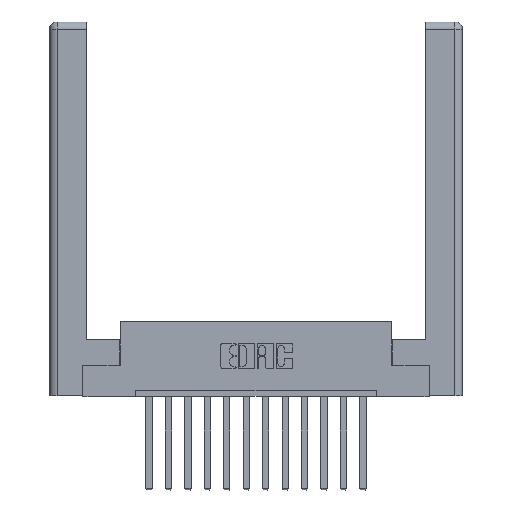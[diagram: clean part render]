
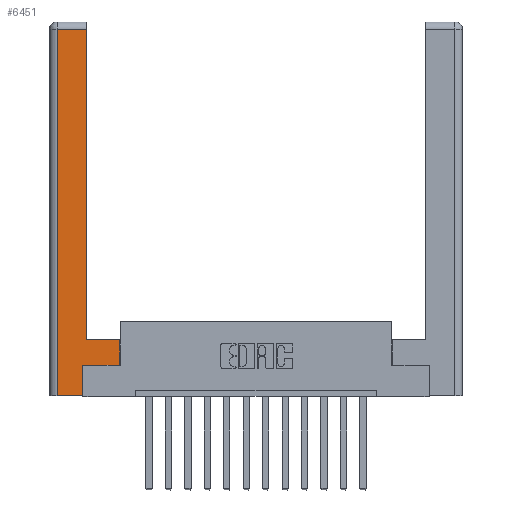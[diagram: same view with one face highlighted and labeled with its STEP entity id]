
A CAD part, top view. The second image highlights one B-rep face of the part: STEP entity #6451.
In plain terms, the highlighted planar face has unit normal (0, 0, 1).
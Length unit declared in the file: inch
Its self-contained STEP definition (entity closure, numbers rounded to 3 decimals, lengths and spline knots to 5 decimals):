
#44 = EDGE_CURVE ( 'NONE', #8756, #13986, #4058, .T. ) ;
#357 = DIRECTION ( 'NONE',  ( -1., 0., 0. ) ) ;
#538 = ORIENTED_EDGE ( 'NONE', *, *, #11361, .T. ) ;
#880 = DIRECTION ( 'NONE',  ( 0., -1., 0. ) ) ;
#919 = CARTESIAN_POINT ( 'NONE',  ( 0.265, 0., 0. ) ) ;
#1040 = VECTOR ( 'NONE', #12653, 39.37008 ) ;
#1096 = VERTEX_POINT ( 'NONE', #3537 ) ;
#1991 = CARTESIAN_POINT ( 'NONE',  ( 0.295, 2.94, 0. ) ) ;
#2086 = EDGE_CURVE ( 'NONE', #8800, #8756, #11748, .T. ) ;
#2091 = LINE ( 'NONE', #3829, #6726 ) ;
#2126 = EDGE_CURVE ( 'NONE', #13986, #3069, #9724, .T. ) ;
#2316 = VECTOR ( 'NONE', #14086, 39.37008 ) ;
#3002 = CARTESIAN_POINT ( 'NONE',  ( 0.0615, 2.94, 0. ) ) ;
#3069 = VERTEX_POINT ( 'NONE', #10200 ) ;
#3183 = ORIENTED_EDGE ( 'NONE', *, *, #6002, .T. ) ;
#3537 = CARTESIAN_POINT ( 'NONE',  ( 0.565, 0.245, 0. ) ) ;
#3702 = VERTEX_POINT ( 'NONE', #1991 ) ;
#3773 = ORIENTED_EDGE ( 'NONE', *, *, #44, .T. ) ;
#3806 = EDGE_CURVE ( 'NONE', #14374, #13888, #2091, .T. ) ;
#3829 = CARTESIAN_POINT ( 'NONE',  ( 0.295, 0.45, 0. ) ) ;
#3985 = PLANE ( 'NONE',  #7229 ) ;
#4058 = LINE ( 'NONE', #919, #9979 ) ;
#4127 = CARTESIAN_POINT ( 'NONE',  ( 0.0615, 0., 0. ) ) ;
#5360 = ORIENTED_EDGE ( 'NONE', *, *, #6466, .T. ) ;
#5579 = ORIENTED_EDGE ( 'NONE', *, *, #2086, .T. ) ;
#5598 = CARTESIAN_POINT ( 'NONE',  ( 0.0615, 0., 0. ) ) ;
#5719 = ORIENTED_EDGE ( 'NONE', *, *, #2126, .T. ) ;
#5774 = DIRECTION ( 'NONE',  ( 1., 0., 0. ) ) ;
#6002 = EDGE_CURVE ( 'NONE', #13888, #3702, #13449, .T. ) ;
#6110 = CARTESIAN_POINT ( 'NONE',  ( 0.565, 0.45, 0. ) ) ;
#6266 = VECTOR ( 'NONE', #14195, 39.37008 ) ;
#6352 = DIRECTION ( 'NONE',  ( 0., 0., -1. ) ) ;
#6451 = ADVANCED_FACE ( 'NONE', ( #6616 ), #3985, .F. ) ;
#6466 = EDGE_CURVE ( 'NONE', #3702, #8800, #12165, .T. ) ;
#6616 = FACE_OUTER_BOUND ( 'NONE', #12034, .T. ) ;
#6726 = VECTOR ( 'NONE', #357, 39.37008 ) ;
#7229 = AXIS2_PLACEMENT_3D ( 'NONE', #11104, #6352, #10031 ) ;
#7402 = DIRECTION ( 'NONE',  ( 0., 1., 0. ) ) ;
#7602 = ORIENTED_EDGE ( 'NONE', *, *, #12802, .T. ) ;
#8293 = CARTESIAN_POINT ( 'NONE',  ( 0.295, 3., 0. ) ) ;
#8756 = VERTEX_POINT ( 'NONE', #4127 ) ;
#8800 = VERTEX_POINT ( 'NONE', #15255 ) ;
#9182 = LINE ( 'NONE', #14432, #9919 ) ;
#9233 = CARTESIAN_POINT ( 'NONE',  ( 0.565, 0.245, 0. ) ) ;
#9724 = LINE ( 'NONE', #12518, #2316 ) ;
#9919 = VECTOR ( 'NONE', #7402, 39.37008 ) ;
#9979 = VECTOR ( 'NONE', #5774, 39.37008 ) ;
#10001 = CARTESIAN_POINT ( 'NONE',  ( 0.265, 0., 0. ) ) ;
#10031 = DIRECTION ( 'NONE',  ( -1., 0., 0. ) ) ;
#10200 = CARTESIAN_POINT ( 'NONE',  ( 0.265, 0.245, 0. ) ) ;
#10500 = CARTESIAN_POINT ( 'NONE',  ( 0.295, 0.45, 0. ) ) ;
#11104 = CARTESIAN_POINT ( 'NONE',  ( 0., 0., 0. ) ) ;
#11361 = EDGE_CURVE ( 'NONE', #1096, #14374, #9182, .T. ) ;
#11748 = LINE ( 'NONE', #5598, #13220 ) ;
#12034 = EDGE_LOOP ( 'NONE', ( #3183, #5360, #5579, #3773, #5719, #7602, #538, #12432 ) ) ;
#12165 = LINE ( 'NONE', #3002, #1040 ) ;
#12432 = ORIENTED_EDGE ( 'NONE', *, *, #3806, .T. ) ;
#12518 = CARTESIAN_POINT ( 'NONE',  ( 0.265, 0.245, 0. ) ) ;
#12653 = DIRECTION ( 'NONE',  ( -1., 0., 0. ) ) ;
#12802 = EDGE_CURVE ( 'NONE', #3069, #1096, #13369, .T. ) ;
#13220 = VECTOR ( 'NONE', #880, 39.37008 ) ;
#13369 = LINE ( 'NONE', #9233, #15014 ) ;
#13449 = LINE ( 'NONE', #8293, #6266 ) ;
#13888 = VERTEX_POINT ( 'NONE', #10500 ) ;
#13974 = DIRECTION ( 'NONE',  ( 1., 0., 0. ) ) ;
#13986 = VERTEX_POINT ( 'NONE', #10001 ) ;
#14086 = DIRECTION ( 'NONE',  ( 0., 1., 0. ) ) ;
#14195 = DIRECTION ( 'NONE',  ( 0., 1., 0. ) ) ;
#14374 = VERTEX_POINT ( 'NONE', #6110 ) ;
#14432 = CARTESIAN_POINT ( 'NONE',  ( 0.565, 0.45, 0. ) ) ;
#15014 = VECTOR ( 'NONE', #13974, 39.37008 ) ;
#15255 = CARTESIAN_POINT ( 'NONE',  ( 0.0615, 2.94, 0. ) ) ;
